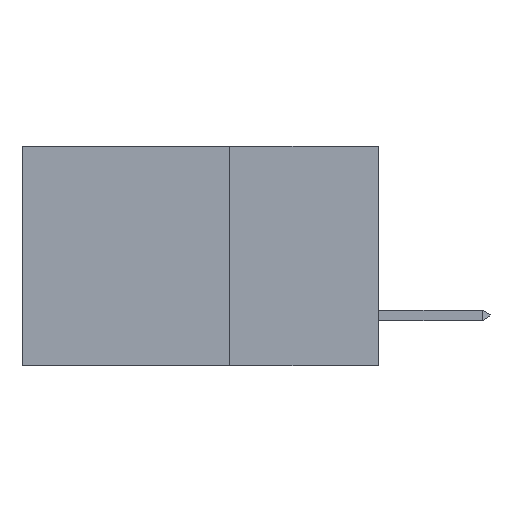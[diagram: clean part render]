
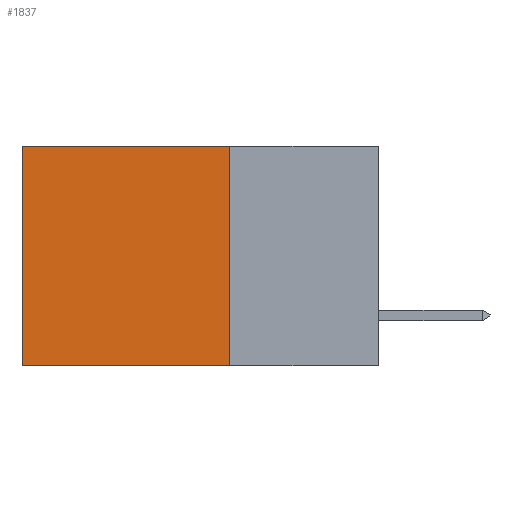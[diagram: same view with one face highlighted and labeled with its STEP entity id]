
A CAD part, left-side view. The second image highlights one B-rep face of the part: STEP entity #1837.
In plain terms, the highlighted planar face has unit normal (-1, 0, 0).
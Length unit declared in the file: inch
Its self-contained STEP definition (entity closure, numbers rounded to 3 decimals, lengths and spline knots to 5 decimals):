
#92 = CARTESIAN_POINT ( 'NONE',  ( 0.2615, 0.25, -0.37 ) ) ;
#153 = DIRECTION ( 'NONE',  ( 1., 0., 0. ) ) ;
#243 = EDGE_CURVE ( 'NONE', #6740, #1318, #8599, .T. ) ;
#853 = ORIENTED_EDGE ( 'NONE', *, *, #243, .T. ) ;
#903 = EDGE_CURVE ( 'NONE', #3782, #6740, #8224, .T. ) ;
#1028 = DIRECTION ( 'NONE',  ( 0., 0., -1. ) ) ;
#1055 = DIRECTION ( 'NONE',  ( 0., 1., 0. ) ) ;
#1318 = VERTEX_POINT ( 'NONE', #10060 ) ;
#1388 = CARTESIAN_POINT ( 'NONE',  ( 0.2615, 0.6, -0.37 ) ) ;
#1776 = EDGE_LOOP ( 'NONE', ( #853, #7888, #9085, #3608 ) ) ;
#1837 = ADVANCED_FACE ( 'NONE', ( #2467 ), #4933, .F. ) ;
#2276 = CARTESIAN_POINT ( 'NONE',  ( 0.2615, 0.25, 0. ) ) ;
#2467 = FACE_OUTER_BOUND ( 'NONE', #1776, .T. ) ;
#2487 = VECTOR ( 'NONE', #1055, 39.37008 ) ;
#3523 = VERTEX_POINT ( 'NONE', #9767 ) ;
#3608 = ORIENTED_EDGE ( 'NONE', *, *, #903, .T. ) ;
#3656 = DIRECTION ( 'NONE',  ( 0., 0., -1. ) ) ;
#3782 = VERTEX_POINT ( 'NONE', #2276 ) ;
#4064 = EDGE_CURVE ( 'NONE', #3782, #3523, #6573, .T. ) ;
#4220 = CARTESIAN_POINT ( 'NONE',  ( 0.2615, 0.25, 0. ) ) ;
#4933 = PLANE ( 'NONE',  #8194 ) ;
#5275 = VECTOR ( 'NONE', #1028, 39.37008 ) ;
#6241 = CARTESIAN_POINT ( 'NONE',  ( 0.2615, 0.25, -0.37 ) ) ;
#6498 = VECTOR ( 'NONE', #7897, 39.37008 ) ;
#6573 = LINE ( 'NONE', #9111, #5275 ) ;
#6740 = VERTEX_POINT ( 'NONE', #6930 ) ;
#6930 = CARTESIAN_POINT ( 'NONE',  ( 0.2615, 0.6, 0. ) ) ;
#7140 = LINE ( 'NONE', #6241, #6498 ) ;
#7888 = ORIENTED_EDGE ( 'NONE', *, *, #9875, .F. ) ;
#7897 = DIRECTION ( 'NONE',  ( 0., 1., 0. ) ) ;
#8194 = AXIS2_PLACEMENT_3D ( 'NONE', #92, #153, #10342 ) ;
#8224 = LINE ( 'NONE', #4220, #2487 ) ;
#8599 = LINE ( 'NONE', #1388, #9589 ) ;
#9085 = ORIENTED_EDGE ( 'NONE', *, *, #4064, .F. ) ;
#9111 = CARTESIAN_POINT ( 'NONE',  ( 0.2615, 0.25, -0.37 ) ) ;
#9589 = VECTOR ( 'NONE', #3656, 39.37008 ) ;
#9767 = CARTESIAN_POINT ( 'NONE',  ( 0.2615, 0.25, -0.37 ) ) ;
#9875 = EDGE_CURVE ( 'NONE', #3523, #1318, #7140, .T. ) ;
#10060 = CARTESIAN_POINT ( 'NONE',  ( 0.2615, 0.6, -0.37 ) ) ;
#10342 = DIRECTION ( 'NONE',  ( 0., 0., -1. ) ) ;
